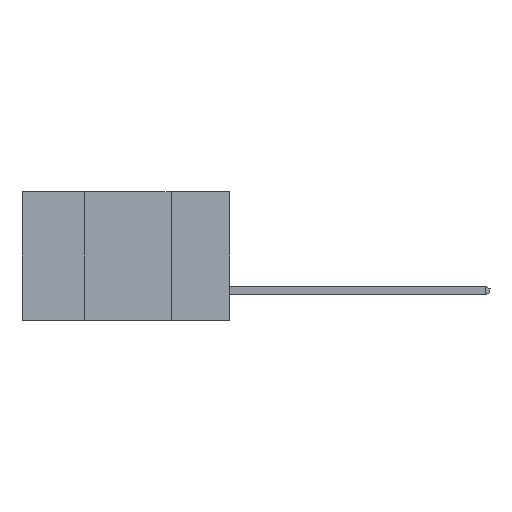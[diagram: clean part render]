
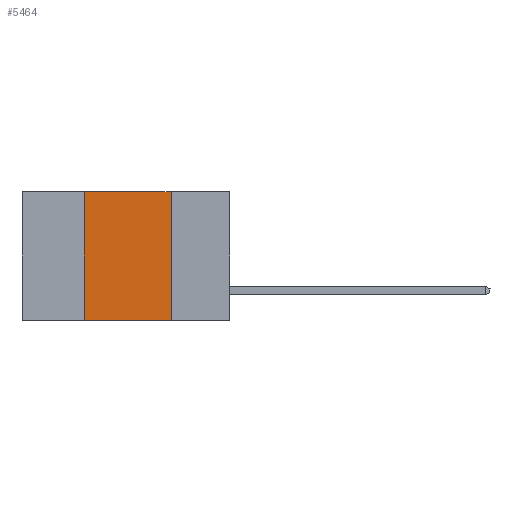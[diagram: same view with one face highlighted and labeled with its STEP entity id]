
A CAD part, left-side view. The second image highlights one B-rep face of the part: STEP entity #5464.
In plain terms, the highlighted planar face has unit normal (-1, 0, 0).
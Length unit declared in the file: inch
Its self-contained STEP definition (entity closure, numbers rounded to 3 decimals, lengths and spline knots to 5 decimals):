
#47 = DIRECTION ( 'NONE',  ( 0., 0., 1. ) ) ;
#629 = VERTEX_POINT ( 'NONE', #6281 ) ;
#935 = DIRECTION ( 'NONE',  ( 0., 0., -1. ) ) ;
#976 = CARTESIAN_POINT ( 'NONE',  ( 0., 0.6, 0. ) ) ;
#1313 = VERTEX_POINT ( 'NONE', #1617 ) ;
#1617 = CARTESIAN_POINT ( 'NONE',  ( 0., 0.17, 0. ) ) ;
#1710 = ORIENTED_EDGE ( 'NONE', *, *, #5205, .F. ) ;
#1720 = ORIENTED_EDGE ( 'NONE', *, *, #3325, .F. ) ;
#1737 = ORIENTED_EDGE ( 'NONE', *, *, #5230, .F. ) ;
#1764 = ORIENTED_EDGE ( 'NONE', *, *, #5340, .T. ) ;
#1996 = CARTESIAN_POINT ( 'NONE',  ( 0., 0.6, 0. ) ) ;
#2132 = VECTOR ( 'NONE', #47, 39.37008 ) ;
#2197 = LINE ( 'NONE', #976, #6527 ) ;
#2252 = VECTOR ( 'NONE', #7876, 39.37008 ) ;
#2803 = DIRECTION ( 'NONE',  ( 0., 0., -1. ) ) ;
#3255 = CARTESIAN_POINT ( 'NONE',  ( 0., 0.17, -0.37 ) ) ;
#3319 = EDGE_LOOP ( 'NONE', ( #1710, #1720, #1737, #1764 ) ) ;
#3325 = EDGE_CURVE ( 'NONE', #629, #1313, #2197, .T. ) ;
#4029 = VERTEX_POINT ( 'NONE', #3255 ) ;
#4334 = LINE ( 'NONE', #7966, #2132 ) ;
#4574 = AXIS2_PLACEMENT_3D ( 'NONE', #1996, #7524, #2803 ) ;
#4795 = DIRECTION ( 'NONE',  ( 0., -1., 0. ) ) ;
#5205 = EDGE_CURVE ( 'NONE', #1313, #4029, #6687, .T. ) ;
#5230 = EDGE_CURVE ( 'NONE', #6477, #629, #4334, .T. ) ;
#5340 = EDGE_CURVE ( 'NONE', #6477, #4029, #6576, .T. ) ;
#5464 = ADVANCED_FACE ( 'NONE', ( #8896 ), #6850, .F. ) ;
#6281 = CARTESIAN_POINT ( 'NONE',  ( 0., 0.42, 0. ) ) ;
#6477 = VERTEX_POINT ( 'NONE', #9582 ) ;
#6527 = VECTOR ( 'NONE', #4795, 39.37008 ) ;
#6576 = LINE ( 'NONE', #9820, #2252 ) ;
#6687 = LINE ( 'NONE', #9242, #8287 ) ;
#6850 = PLANE ( 'NONE',  #4574 ) ;
#7524 = DIRECTION ( 'NONE',  ( 1., 0., 0. ) ) ;
#7876 = DIRECTION ( 'NONE',  ( 0., -1., 0. ) ) ;
#7966 = CARTESIAN_POINT ( 'NONE',  ( 0., 0.42, 0. ) ) ;
#8287 = VECTOR ( 'NONE', #935, 39.37008 ) ;
#8896 = FACE_OUTER_BOUND ( 'NONE', #3319, .T. ) ;
#9242 = CARTESIAN_POINT ( 'NONE',  ( 0., 0.17, 0. ) ) ;
#9582 = CARTESIAN_POINT ( 'NONE',  ( 0., 0.42, -0.37 ) ) ;
#9820 = CARTESIAN_POINT ( 'NONE',  ( 0., 0.6, -0.37 ) ) ;
